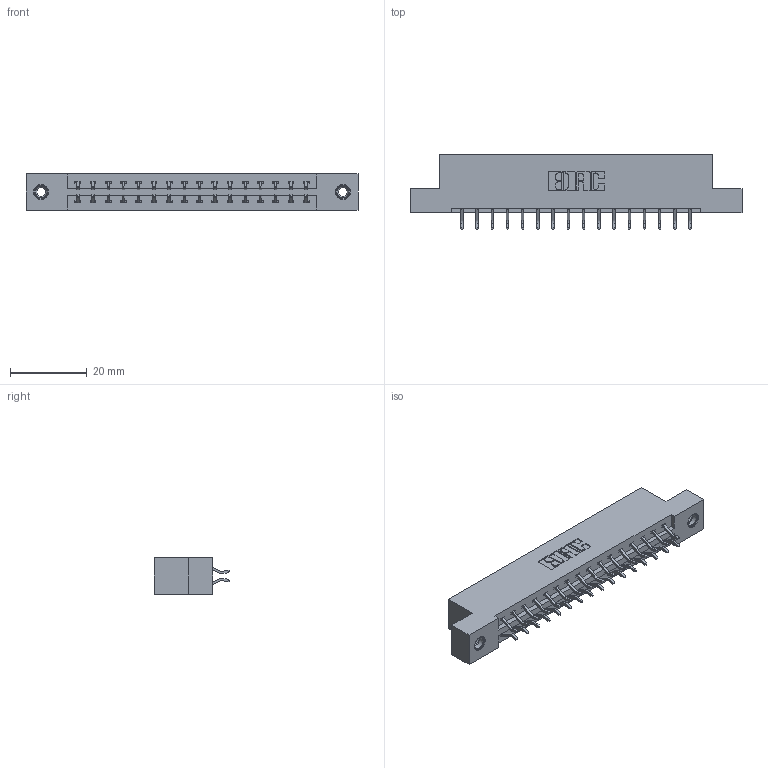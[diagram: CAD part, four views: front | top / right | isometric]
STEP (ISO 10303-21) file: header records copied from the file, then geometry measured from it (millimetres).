
FILE_DESCRIPTION (( 'STEP AP203' ), '1' );
FILE_NAME ('337-032-556-208.STEP', '2019-10-08T19:37:10', ( '' ), ( '' ), 'SwSTEP 2.0', 'SolidWorks 2016', '' );
FILE_SCHEMA (( 'CONFIG_CONTROL_DESIGN' ));
Length unit declared in the file: inch
Products named in the file (4): 337 Part_Flush Mounting Lugs - 0.156 Dia-TI; 345-292-001_556 Tail; 337-032-556-208; 345-250-001_345-250-003-102
Assembly tree (35 placements, depth 2):
  337-032-556-208
    337 Part_Flush Mounting Lugs - 0.156 Dia-TI
    345-292-001_556 Tail  x32
    345-250-001_345-250-003-102  x2
Bounding box: 86.41 x 19.57 x 9.4 mm (x, y, z)
Volume: 8752.8 mm3; surface area: 9632.6 mm2
Topology: 35 solids, 35 shells, 2094 faces, 6175 edges, 4066 vertices
Faces by surface type: plane 1446, cylinder 632, cone 12, torus 4
Entity records: 17174 total; most frequent: CARTESIAN_POINT 2909, ORIENTED_EDGE 2826, DIRECTION 2543, EDGE_CURVE 1413, VECTOR 1257, LINE 1257, VERTEX_POINT 936, AXIS2_PLACEMENT_3D 643
